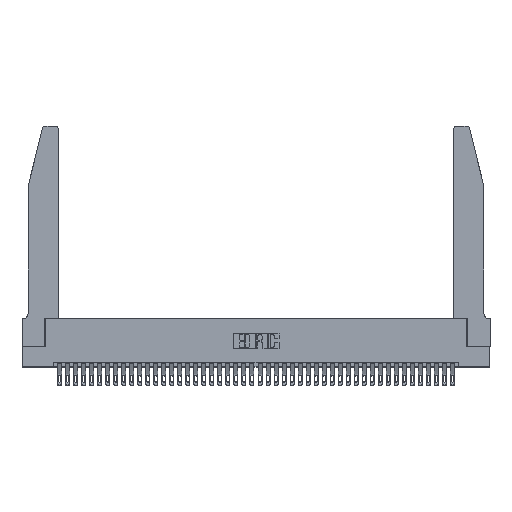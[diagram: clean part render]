
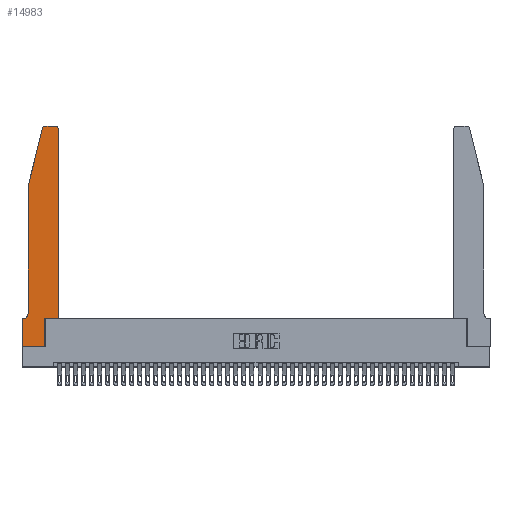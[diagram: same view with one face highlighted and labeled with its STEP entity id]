
A CAD part, top view. The second image highlights one B-rep face of the part: STEP entity #14983.
In plain terms, the highlighted planar face has unit normal (0, 0, 1).
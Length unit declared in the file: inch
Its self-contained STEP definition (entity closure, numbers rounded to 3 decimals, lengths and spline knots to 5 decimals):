
#233 = VERTEX_POINT ( 'NONE', #42486 ) ;
#408 = VECTOR ( 'NONE', #3334, 39.37008 ) ;
#560 = ORIENTED_EDGE ( 'NONE', *, *, #19638, .T. ) ;
#1002 = EDGE_CURVE ( 'NONE', #41501, #19359, #9263, .T. ) ;
#1079 = ORIENTED_EDGE ( 'NONE', *, *, #23188, .T. ) ;
#1343 = VERTEX_POINT ( 'NONE', #42698 ) ;
#1481 = CARTESIAN_POINT ( 'NONE',  ( 0., 0.35, 0.37 ) ) ;
#1711 = CARTESIAN_POINT ( 'NONE',  ( 0.0055, 0.35, 0.37 ) ) ;
#2303 = LINE ( 'NONE', #28065, #36811 ) ;
#3334 = DIRECTION ( 'NONE',  ( 1., 0., 0. ) ) ;
#3727 = AXIS2_PLACEMENT_3D ( 'NONE', #1481, #18471, #41596 ) ;
#3779 = ORIENTED_EDGE ( 'NONE', *, *, #23762, .T. ) ;
#3918 = CARTESIAN_POINT ( 'NONE',  ( 0.0755, 2., 0.37 ) ) ;
#5341 = VECTOR ( 'NONE', #13971, 39.37008 ) ;
#5627 = LINE ( 'NONE', #10258, #13570 ) ;
#5786 = CARTESIAN_POINT ( 'NONE',  ( 0.4505, 0.35, 0.37 ) ) ;
#6472 = ORIENTED_EDGE ( 'NONE', *, *, #13203, .T. ) ;
#6531 = EDGE_LOOP ( 'NONE', ( #3779, #32519, #7000, #1079, #37716, #29956, #38742, #23215, #6472, #41835, #560, #27395 ) ) ;
#6713 = AXIS2_PLACEMENT_3D ( 'NONE', #33316, #13441, #36626 ) ;
#6847 = VECTOR ( 'NONE', #13275, 39.37008 ) ;
#7000 = ORIENTED_EDGE ( 'NONE', *, *, #31000, .T. ) ;
#9263 = CIRCLE ( 'NONE', #27290, 0.07 ) ;
#9416 = CARTESIAN_POINT ( 'NONE',  ( 0.4505, 2.72, 0.37 ) ) ;
#9497 = LINE ( 'NONE', #26776, #408 ) ;
#10111 = VECTOR ( 'NONE', #24871, 39.37008 ) ;
#10258 = CARTESIAN_POINT ( 'NONE',  ( 0.0755, 2., 0.37 ) ) ;
#10487 = CARTESIAN_POINT ( 'NONE',  ( 0.25487, 2.72718, 0.37 ) ) ;
#10825 = CARTESIAN_POINT ( 'NONE',  ( 0.0055, 0.42, 0.37 ) ) ;
#10865 = EDGE_CURVE ( 'NONE', #38407, #38288, #9497, .T. ) ;
#10988 = EDGE_CURVE ( 'NONE', #15261, #37863, #39629, .T. ) ;
#11166 = LINE ( 'NONE', #38060, #10111 ) ;
#11418 = LINE ( 'NONE', #42862, #20319 ) ;
#13203 = EDGE_CURVE ( 'NONE', #38288, #24157, #19238, .T. ) ;
#13215 = CARTESIAN_POINT ( 'NONE',  ( 0.284, 2.75, 0.37 ) ) ;
#13275 = DIRECTION ( 'NONE',  ( 1., 0., 0. ) ) ;
#13441 = DIRECTION ( 'NONE',  ( 0., 0., 1. ) ) ;
#13570 = VECTOR ( 'NONE', #17495, 39.37008 ) ;
#13971 = DIRECTION ( 'NONE',  ( 0., -1., 0. ) ) ;
#14136 = CARTESIAN_POINT ( 'NONE',  ( 0.284, 2.72, 0.37 ) ) ;
#14225 = DIRECTION ( 'NONE',  ( -1., 0., 0. ) ) ;
#14983 = ADVANCED_FACE ( 'NONE', ( #20133 ), #38306, .T. ) ;
#15261 = VERTEX_POINT ( 'NONE', #13215 ) ;
#15791 = LINE ( 'NONE', #23146, #6847 ) ;
#17478 = DIRECTION ( 'NONE',  ( 1., 0., 0. ) ) ;
#17495 = DIRECTION ( 'NONE',  ( 0., -1., 0. ) ) ;
#18471 = DIRECTION ( 'NONE',  ( 0., 0., 1. ) ) ;
#18896 = VERTEX_POINT ( 'NONE', #5786 ) ;
#19238 = LINE ( 'NONE', #38739, #28064 ) ;
#19359 = VERTEX_POINT ( 'NONE', #1711 ) ;
#19638 = EDGE_CURVE ( 'NONE', #18896, #34762, #11166, .T. ) ;
#19723 = DIRECTION ( 'NONE',  ( -1., 0., 0. ) ) ;
#19951 = CARTESIAN_POINT ( 'NONE',  ( 0., 0., 0.37 ) ) ;
#20133 = FACE_OUTER_BOUND ( 'NONE', #6531, .T. ) ;
#20319 = VECTOR ( 'NONE', #19723, 39.37008 ) ;
#21329 = EDGE_CURVE ( 'NONE', #34762, #233, #41173, .T. ) ;
#23146 = CARTESIAN_POINT ( 'NONE',  ( 0.4505, 0.35, 0.37 ) ) ;
#23188 = EDGE_CURVE ( 'NONE', #29282, #41501, #5627, .T. ) ;
#23215 = ORIENTED_EDGE ( 'NONE', *, *, #10865, .T. ) ;
#23762 = EDGE_CURVE ( 'NONE', #233, #15261, #11418, .T. ) ;
#24157 = VERTEX_POINT ( 'NONE', #28247 ) ;
#24629 = EDGE_CURVE ( 'NONE', #19359, #1343, #2303, .T. ) ;
#24871 = DIRECTION ( 'NONE',  ( 0., 1., 0. ) ) ;
#26776 = CARTESIAN_POINT ( 'NONE',  ( 0., 0., 0.37 ) ) ;
#26820 = EDGE_CURVE ( 'NONE', #1343, #38407, #31967, .T. ) ;
#27290 = AXIS2_PLACEMENT_3D ( 'NONE', #10825, #34103, #14225 ) ;
#27395 = ORIENTED_EDGE ( 'NONE', *, *, #21329, .T. ) ;
#28064 = VECTOR ( 'NONE', #42032, 39.37008 ) ;
#28065 = CARTESIAN_POINT ( 'NONE',  ( 0.0755, 0.35, 0.37 ) ) ;
#28247 = CARTESIAN_POINT ( 'NONE',  ( 0.2865, 0.35, 0.37 ) ) ;
#29282 = VERTEX_POINT ( 'NONE', #35113 ) ;
#29415 = AXIS2_PLACEMENT_3D ( 'NONE', #14136, #37318, #17478 ) ;
#29956 = ORIENTED_EDGE ( 'NONE', *, *, #24629, .T. ) ;
#31000 = EDGE_CURVE ( 'NONE', #37863, #29282, #32305, .T. ) ;
#31967 = LINE ( 'NONE', #37155, #5341 ) ;
#32305 = LINE ( 'NONE', #3918, #40062 ) ;
#32519 = ORIENTED_EDGE ( 'NONE', *, *, #10988, .T. ) ;
#32552 = CARTESIAN_POINT ( 'NONE',  ( 0.2865, 0., 0.37 ) ) ;
#33316 = CARTESIAN_POINT ( 'NONE',  ( 0.4205, 2.72, 0.37 ) ) ;
#33999 = DIRECTION ( 'NONE',  ( -0.239, -0.971, 0. ) ) ;
#34103 = DIRECTION ( 'NONE',  ( 0., 0., -1. ) ) ;
#34762 = VERTEX_POINT ( 'NONE', #9416 ) ;
#35113 = CARTESIAN_POINT ( 'NONE',  ( 0.0755, 2., 0.37 ) ) ;
#36626 = DIRECTION ( 'NONE',  ( 1., 0., 0. ) ) ;
#36811 = VECTOR ( 'NONE', #38614, 39.37008 ) ;
#36821 = EDGE_CURVE ( 'NONE', #24157, #18896, #15791, .T. ) ;
#37155 = CARTESIAN_POINT ( 'NONE',  ( 0., 0., 0.37 ) ) ;
#37318 = DIRECTION ( 'NONE',  ( 0., 0., 1. ) ) ;
#37716 = ORIENTED_EDGE ( 'NONE', *, *, #1002, .T. ) ;
#37863 = VERTEX_POINT ( 'NONE', #10487 ) ;
#37900 = CARTESIAN_POINT ( 'NONE',  ( 0.0755, 0.42, 0.37 ) ) ;
#38060 = CARTESIAN_POINT ( 'NONE',  ( 0.4505, 0.35, 0.37 ) ) ;
#38288 = VERTEX_POINT ( 'NONE', #32552 ) ;
#38306 = PLANE ( 'NONE',  #3727 ) ;
#38407 = VERTEX_POINT ( 'NONE', #19951 ) ;
#38614 = DIRECTION ( 'NONE',  ( -1., 0., 0. ) ) ;
#38739 = CARTESIAN_POINT ( 'NONE',  ( 0.2865, 0.35, 0.37 ) ) ;
#38742 = ORIENTED_EDGE ( 'NONE', *, *, #26820, .T. ) ;
#39629 = CIRCLE ( 'NONE', #29415, 0.03 ) ;
#40062 = VECTOR ( 'NONE', #33999, 39.37008 ) ;
#41173 = CIRCLE ( 'NONE', #6713, 0.03 ) ;
#41501 = VERTEX_POINT ( 'NONE', #37900 ) ;
#41596 = DIRECTION ( 'NONE',  ( 1., 0., 0. ) ) ;
#41835 = ORIENTED_EDGE ( 'NONE', *, *, #36821, .T. ) ;
#42032 = DIRECTION ( 'NONE',  ( 0., 1., 0. ) ) ;
#42486 = CARTESIAN_POINT ( 'NONE',  ( 0.4205, 2.75, 0.37 ) ) ;
#42698 = CARTESIAN_POINT ( 'NONE',  ( 0., 0.35, 0.37 ) ) ;
#42862 = CARTESIAN_POINT ( 'NONE',  ( 0.2605, 2.75, 0.37 ) ) ;
